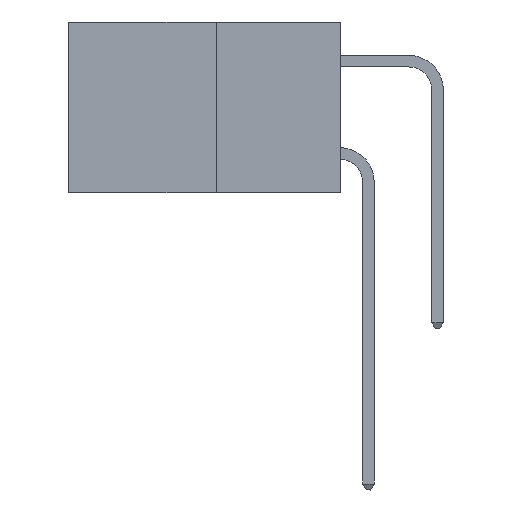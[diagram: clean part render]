
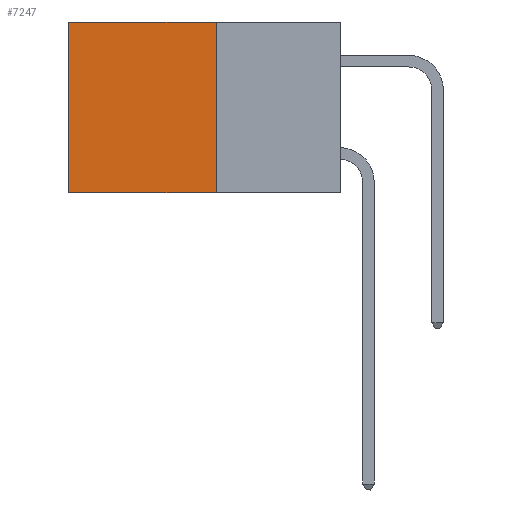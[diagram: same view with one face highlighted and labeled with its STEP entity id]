
A CAD part, left-side view. The second image highlights one B-rep face of the part: STEP entity #7247.
In plain terms, the highlighted planar face has unit normal (-1, 0, 0).
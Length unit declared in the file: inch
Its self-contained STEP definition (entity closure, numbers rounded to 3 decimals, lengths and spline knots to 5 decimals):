
#94 = VERTEX_POINT ( 'NONE', #2922 ) ;
#260 = FACE_OUTER_BOUND ( 'NONE', #6675, .T. ) ;
#390 = LINE ( 'NONE', #8182, #4585 ) ;
#414 = DIRECTION ( 'NONE',  ( 0., 0., -1. ) ) ;
#785 = EDGE_CURVE ( 'NONE', #5999, #5359, #3741, .T. ) ;
#1465 = CARTESIAN_POINT ( 'NONE',  ( 0.277, 0.27, 0. ) ) ;
#2055 = PLANE ( 'NONE',  #5185 ) ;
#2267 = VECTOR ( 'NONE', #5617, 39.37008 ) ;
#2922 = CARTESIAN_POINT ( 'NONE',  ( 0.277, 0.59, -0.37 ) ) ;
#3084 = CARTESIAN_POINT ( 'NONE',  ( 0.277, 0.59, 0. ) ) ;
#3513 = LINE ( 'NONE', #4349, #7394 ) ;
#3741 = LINE ( 'NONE', #7166, #9265 ) ;
#3873 = DIRECTION ( 'NONE',  ( 0., 1., 0. ) ) ;
#4098 = EDGE_CURVE ( 'NONE', #5999, #7802, #3513, .T. ) ;
#4336 = EDGE_CURVE ( 'NONE', #7802, #94, #6663, .T. ) ;
#4349 = CARTESIAN_POINT ( 'NONE',  ( 0.277, 0.27, 0. ) ) ;
#4585 = VECTOR ( 'NONE', #8809, 39.37008 ) ;
#4594 = CARTESIAN_POINT ( 'NONE',  ( 0.277, 0.27, -0.37 ) ) ;
#5154 = ORIENTED_EDGE ( 'NONE', *, *, #785, .F. ) ;
#5185 = AXIS2_PLACEMENT_3D ( 'NONE', #4594, #5456, #414 ) ;
#5359 = VERTEX_POINT ( 'NONE', #8643 ) ;
#5456 = DIRECTION ( 'NONE',  ( 1., 0., 0. ) ) ;
#5617 = DIRECTION ( 'NONE',  ( 0., 0., -1. ) ) ;
#5655 = CARTESIAN_POINT ( 'NONE',  ( 0.277, 0.59, -0.37 ) ) ;
#5787 = EDGE_CURVE ( 'NONE', #5359, #94, #390, .T. ) ;
#5938 = ORIENTED_EDGE ( 'NONE', *, *, #5787, .F. ) ;
#5999 = VERTEX_POINT ( 'NONE', #1465 ) ;
#6663 = LINE ( 'NONE', #5655, #2267 ) ;
#6675 = EDGE_LOOP ( 'NONE', ( #7493, #5938, #5154, #8873 ) ) ;
#7166 = CARTESIAN_POINT ( 'NONE',  ( 0.277, 0.27, -0.37 ) ) ;
#7247 = ADVANCED_FACE ( 'NONE', ( #260 ), #2055, .F. ) ;
#7394 = VECTOR ( 'NONE', #3873, 39.37008 ) ;
#7493 = ORIENTED_EDGE ( 'NONE', *, *, #4336, .T. ) ;
#7802 = VERTEX_POINT ( 'NONE', #3084 ) ;
#8182 = CARTESIAN_POINT ( 'NONE',  ( 0.277, 0.27, -0.37 ) ) ;
#8643 = CARTESIAN_POINT ( 'NONE',  ( 0.277, 0.27, -0.37 ) ) ;
#8809 = DIRECTION ( 'NONE',  ( 0., 1., 0. ) ) ;
#8873 = ORIENTED_EDGE ( 'NONE', *, *, #4098, .T. ) ;
#9263 = DIRECTION ( 'NONE',  ( 0., 0., -1. ) ) ;
#9265 = VECTOR ( 'NONE', #9263, 39.37008 ) ;
